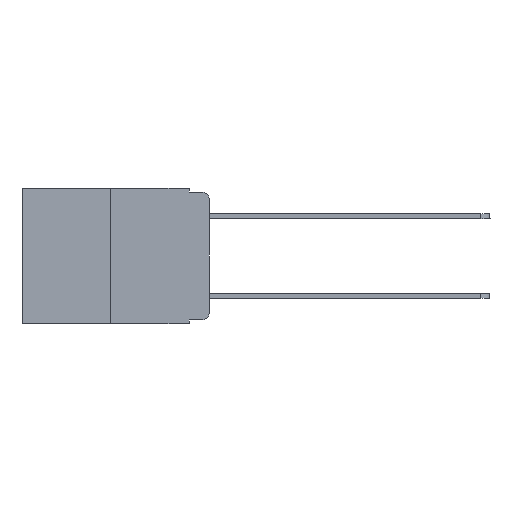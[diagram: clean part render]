
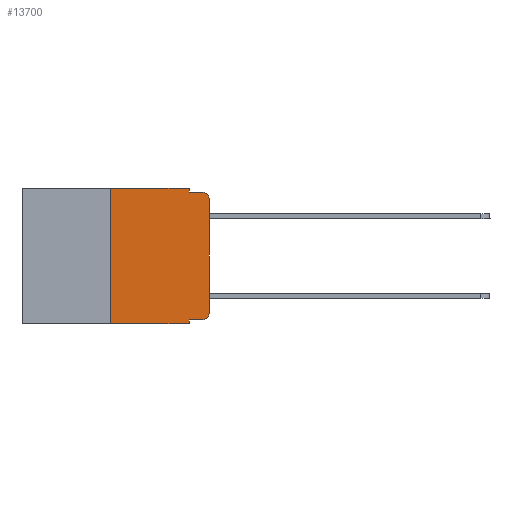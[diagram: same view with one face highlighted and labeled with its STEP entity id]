
A CAD part, left-side view. The second image highlights one B-rep face of the part: STEP entity #13700.
In plain terms, the highlighted planar face has unit normal (-1, 0, 0).
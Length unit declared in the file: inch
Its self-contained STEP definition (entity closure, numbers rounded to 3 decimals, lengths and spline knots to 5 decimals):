
#90 = VECTOR ( 'NONE', #13740, 39.37008 ) ;
#174 = CARTESIAN_POINT ( 'NONE',  ( 0., 0.25, 0. ) ) ;
#437 = CARTESIAN_POINT ( 'NONE',  ( 0., 0.25, 0. ) ) ;
#473 = VERTEX_POINT ( 'NONE', #1929 ) ;
#694 = ORIENTED_EDGE ( 'NONE', *, *, #14351, .T. ) ;
#785 = VECTOR ( 'NONE', #6273, 39.37008 ) ;
#819 = DIRECTION ( 'NONE',  ( 0., 0., -1. ) ) ;
#943 = CARTESIAN_POINT ( 'NONE',  ( 0., 0.02, -0.03 ) ) ;
#1017 = DIRECTION ( 'NONE',  ( -1., 0., 0. ) ) ;
#1388 = VERTEX_POINT ( 'NONE', #6953 ) ;
#1594 = AXIS2_PLACEMENT_3D ( 'NONE', #4846, #16992, #14204 ) ;
#1929 = CARTESIAN_POINT ( 'NONE',  ( 0., 0., -0.313 ) ) ;
#1977 = LINE ( 'NONE', #14237, #17415 ) ;
#2135 = CIRCLE ( 'NONE', #5966, 0.02 ) ;
#2567 = ORIENTED_EDGE ( 'NONE', *, *, #4928, .F. ) ;
#2585 = ORIENTED_EDGE ( 'NONE', *, *, #15867, .F. ) ;
#2624 = VECTOR ( 'NONE', #13058, 39.37008 ) ;
#2794 = VECTOR ( 'NONE', #11058, 39.37008 ) ;
#3030 = CARTESIAN_POINT ( 'NONE',  ( 0., 0.051, -0.01 ) ) ;
#3083 = CARTESIAN_POINT ( 'NONE',  ( 0., 0.051, -0.01 ) ) ;
#3752 = DIRECTION ( 'NONE',  ( 0., 0., -1. ) ) ;
#3913 = CARTESIAN_POINT ( 'NONE',  ( 0., 0.02, -0.313 ) ) ;
#4035 = VERTEX_POINT ( 'NONE', #3030 ) ;
#4194 = VERTEX_POINT ( 'NONE', #6424 ) ;
#4297 = EDGE_CURVE ( 'NONE', #19101, #473, #2135, .T. ) ;
#4564 = ORIENTED_EDGE ( 'NONE', *, *, #4568, .T. ) ;
#4568 = EDGE_CURVE ( 'NONE', #15684, #19101, #1977, .T. ) ;
#4786 = LINE ( 'NONE', #3083, #19379 ) ;
#4846 = CARTESIAN_POINT ( 'NONE',  ( 0., 0.473, 0. ) ) ;
#4928 = EDGE_CURVE ( 'NONE', #12361, #1388, #12812, .T. ) ;
#5257 = CARTESIAN_POINT ( 'NONE',  ( 0., 0.473, 0. ) ) ;
#5269 = LINE ( 'NONE', #12915, #6810 ) ;
#5680 = ORIENTED_EDGE ( 'NONE', *, *, #4297, .T. ) ;
#5966 = AXIS2_PLACEMENT_3D ( 'NONE', #3913, #1017, #819 ) ;
#6273 = DIRECTION ( 'NONE',  ( 0., 0., 1. ) ) ;
#6424 = CARTESIAN_POINT ( 'NONE',  ( 0., 0., -0.03 ) ) ;
#6808 = LINE ( 'NONE', #9921, #9614 ) ;
#6810 = VECTOR ( 'NONE', #9963, 39.37008 ) ;
#6953 = CARTESIAN_POINT ( 'NONE',  ( 0., 0.051, 0. ) ) ;
#7010 = LINE ( 'NONE', #18965, #2624 ) ;
#7492 = LINE ( 'NONE', #174, #785 ) ;
#7796 = DIRECTION ( 'NONE',  ( 0., -1., 0. ) ) ;
#7901 = ORIENTED_EDGE ( 'NONE', *, *, #12078, .T. ) ;
#8147 = CIRCLE ( 'NONE', #16061, 0.02 ) ;
#8374 = DIRECTION ( 'NONE',  ( 0., -1., 0. ) ) ;
#8846 = EDGE_CURVE ( 'NONE', #4035, #11198, #4786, .T. ) ;
#9167 = ORIENTED_EDGE ( 'NONE', *, *, #13248, .F. ) ;
#9237 = EDGE_LOOP ( 'NONE', ( #7901, #13084, #9375, #15163, #2567, #9167, #694, #2585, #4564, #5680 ) ) ;
#9375 = ORIENTED_EDGE ( 'NONE', *, *, #8846, .F. ) ;
#9614 = VECTOR ( 'NONE', #15958, 39.37008 ) ;
#9921 = CARTESIAN_POINT ( 'NONE',  ( 0., 0.473, -0.343 ) ) ;
#9963 = DIRECTION ( 'NONE',  ( 0., 0., 1. ) ) ;
#11058 = DIRECTION ( 'NONE',  ( 0., -1., 0. ) ) ;
#11198 = VERTEX_POINT ( 'NONE', #11696 ) ;
#11347 = DIRECTION ( 'NONE',  ( -1., 0., 0. ) ) ;
#11696 = CARTESIAN_POINT ( 'NONE',  ( 0., 0.02, -0.01 ) ) ;
#12078 = EDGE_CURVE ( 'NONE', #473, #4194, #5269, .T. ) ;
#12113 = VERTEX_POINT ( 'NONE', #14706 ) ;
#12168 = CARTESIAN_POINT ( 'NONE',  ( 0., 0.051, 0. ) ) ;
#12361 = VERTEX_POINT ( 'NONE', #437 ) ;
#12412 = FACE_OUTER_BOUND ( 'NONE', #9237, .T. ) ;
#12486 = CARTESIAN_POINT ( 'NONE',  ( 0., 0.051, -0.333 ) ) ;
#12812 = LINE ( 'NONE', #5257, #2794 ) ;
#12915 = CARTESIAN_POINT ( 'NONE',  ( 0., 0., 0. ) ) ;
#13024 = CARTESIAN_POINT ( 'NONE',  ( 0., 0.02, -0.333 ) ) ;
#13058 = DIRECTION ( 'NONE',  ( 0., 0., -1. ) ) ;
#13084 = ORIENTED_EDGE ( 'NONE', *, *, #18287, .T. ) ;
#13248 = EDGE_CURVE ( 'NONE', #16638, #12361, #7492, .T. ) ;
#13700 = ADVANCED_FACE ( 'NONE', ( #12412 ), #18698, .F. ) ;
#13740 = DIRECTION ( 'NONE',  ( 0., 0., -1. ) ) ;
#14204 = DIRECTION ( 'NONE',  ( 0., 0., -1. ) ) ;
#14237 = CARTESIAN_POINT ( 'NONE',  ( 0., 0.051, -0.333 ) ) ;
#14351 = EDGE_CURVE ( 'NONE', #16638, #12113, #6808, .T. ) ;
#14706 = CARTESIAN_POINT ( 'NONE',  ( 0., 0.051, -0.343 ) ) ;
#15163 = ORIENTED_EDGE ( 'NONE', *, *, #16048, .F. ) ;
#15684 = VERTEX_POINT ( 'NONE', #12486 ) ;
#15867 = EDGE_CURVE ( 'NONE', #15684, #12113, #7010, .T. ) ;
#15958 = DIRECTION ( 'NONE',  ( 0., -1., 0. ) ) ;
#16048 = EDGE_CURVE ( 'NONE', #1388, #4035, #19676, .T. ) ;
#16061 = AXIS2_PLACEMENT_3D ( 'NONE', #943, #11347, #3752 ) ;
#16638 = VERTEX_POINT ( 'NONE', #16826 ) ;
#16826 = CARTESIAN_POINT ( 'NONE',  ( 0., 0.25, -0.343 ) ) ;
#16992 = DIRECTION ( 'NONE',  ( 1., 0., 0. ) ) ;
#17415 = VECTOR ( 'NONE', #8374, 39.37008 ) ;
#18287 = EDGE_CURVE ( 'NONE', #4194, #11198, #8147, .T. ) ;
#18698 = PLANE ( 'NONE',  #1594 ) ;
#18965 = CARTESIAN_POINT ( 'NONE',  ( 0., 0.051, 0. ) ) ;
#19101 = VERTEX_POINT ( 'NONE', #13024 ) ;
#19379 = VECTOR ( 'NONE', #7796, 39.37008 ) ;
#19676 = LINE ( 'NONE', #12168, #90 ) ;
